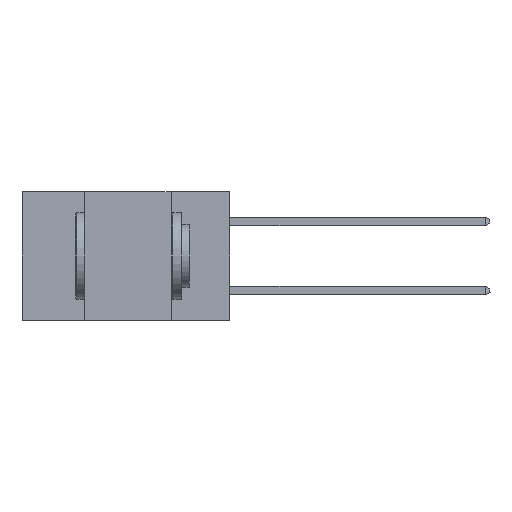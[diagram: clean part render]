
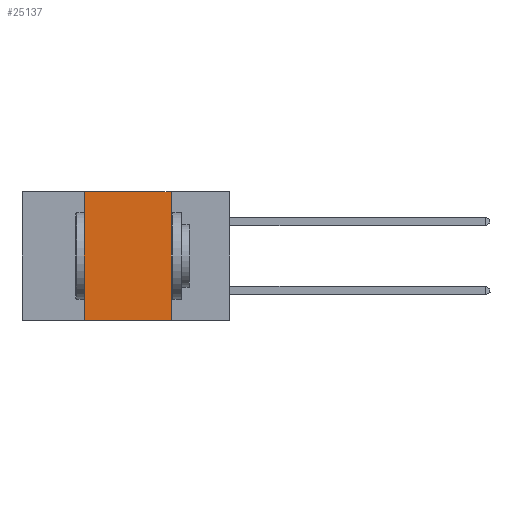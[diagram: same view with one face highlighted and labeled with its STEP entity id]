
A CAD part, left-side view. The second image highlights one B-rep face of the part: STEP entity #25137.
In plain terms, the highlighted planar face has unit normal (-1, 0, 0).
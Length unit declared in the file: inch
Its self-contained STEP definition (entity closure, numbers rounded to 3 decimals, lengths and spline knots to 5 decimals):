
#104 = CARTESIAN_POINT ( 'NONE',  ( 0., 0.6, 0. ) ) ;
#217 = VERTEX_POINT ( 'NONE', #31177 ) ;
#833 = ORIENTED_EDGE ( 'NONE', *, *, #16557, .F. ) ;
#921 = LINE ( 'NONE', #16515, #22176 ) ;
#1629 = PLANE ( 'NONE',  #20739 ) ;
#2752 = VERTEX_POINT ( 'NONE', #32776 ) ;
#2958 = EDGE_CURVE ( 'NONE', #5258, #217, #5326, .T. ) ;
#5258 = VERTEX_POINT ( 'NONE', #13636 ) ;
#5326 = LINE ( 'NONE', #104, #11769 ) ;
#6043 = VECTOR ( 'NONE', #14849, 39.37008 ) ;
#7350 = ORIENTED_EDGE ( 'NONE', *, *, #2958, .F. ) ;
#9101 = CARTESIAN_POINT ( 'NONE',  ( 0., 0.42, -0.37 ) ) ;
#9663 = CARTESIAN_POINT ( 'NONE',  ( 0., 0.6, -0.37 ) ) ;
#9708 = DIRECTION ( 'NONE',  ( 1., 0., 0. ) ) ;
#9851 = EDGE_CURVE ( 'NONE', #33708, #2752, #11372, .T. ) ;
#11372 = LINE ( 'NONE', #9663, #25731 ) ;
#11769 = VECTOR ( 'NONE', #15403, 39.37008 ) ;
#12255 = DIRECTION ( 'NONE',  ( 0., 0., -1. ) ) ;
#13363 = DIRECTION ( 'NONE',  ( 0., 0., -1. ) ) ;
#13636 = CARTESIAN_POINT ( 'NONE',  ( 0., 0.42, 0. ) ) ;
#14849 = DIRECTION ( 'NONE',  ( 0., 0., 1. ) ) ;
#15403 = DIRECTION ( 'NONE',  ( 0., -1., 0. ) ) ;
#16515 = CARTESIAN_POINT ( 'NONE',  ( 0., 0.17, 0. ) ) ;
#16557 = EDGE_CURVE ( 'NONE', #217, #2752, #921, .T. ) ;
#17571 = EDGE_LOOP ( 'NONE', ( #833, #7350, #31831, #30642 ) ) ;
#18627 = EDGE_CURVE ( 'NONE', #33708, #5258, #26904, .T. ) ;
#20739 = AXIS2_PLACEMENT_3D ( 'NONE', #25436, #9708, #12255 ) ;
#22175 = CARTESIAN_POINT ( 'NONE',  ( 0., 0.42, 0. ) ) ;
#22176 = VECTOR ( 'NONE', #13363, 39.37008 ) ;
#22745 = DIRECTION ( 'NONE',  ( 0., -1., 0. ) ) ;
#24793 = FACE_OUTER_BOUND ( 'NONE', #17571, .T. ) ;
#25137 = ADVANCED_FACE ( 'NONE', ( #24793 ), #1629, .F. ) ;
#25436 = CARTESIAN_POINT ( 'NONE',  ( 0., 0.6, 0. ) ) ;
#25731 = VECTOR ( 'NONE', #22745, 39.37008 ) ;
#26904 = LINE ( 'NONE', #22175, #6043 ) ;
#30642 = ORIENTED_EDGE ( 'NONE', *, *, #9851, .T. ) ;
#31177 = CARTESIAN_POINT ( 'NONE',  ( 0., 0.17, 0. ) ) ;
#31831 = ORIENTED_EDGE ( 'NONE', *, *, #18627, .F. ) ;
#32776 = CARTESIAN_POINT ( 'NONE',  ( 0., 0.17, -0.37 ) ) ;
#33708 = VERTEX_POINT ( 'NONE', #9101 ) ;
